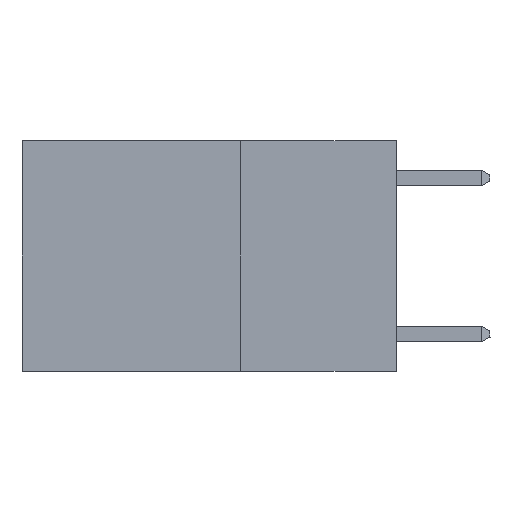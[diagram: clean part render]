
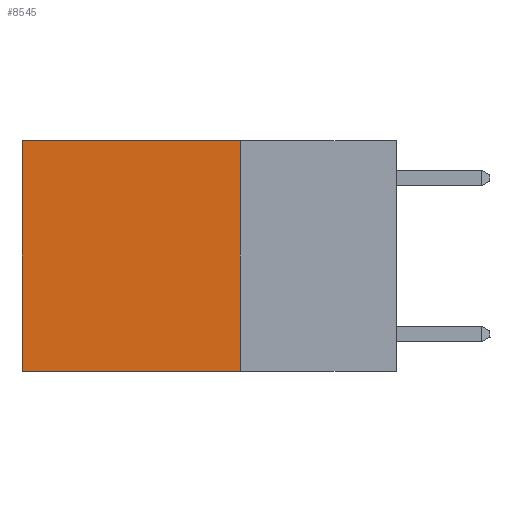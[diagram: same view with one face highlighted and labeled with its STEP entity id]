
A CAD part, left-side view. The second image highlights one B-rep face of the part: STEP entity #8545.
In plain terms, the highlighted planar face has unit normal (-1, 0, 0).
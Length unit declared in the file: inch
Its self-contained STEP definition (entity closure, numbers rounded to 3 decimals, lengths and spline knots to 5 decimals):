
#135 = LINE ( 'NONE', #8784, #15223 ) ;
#398 = CARTESIAN_POINT ( 'NONE',  ( 0.2625, 0.25, 0. ) ) ;
#1139 = CARTESIAN_POINT ( 'NONE',  ( 0.2625, 0.25, -0.37 ) ) ;
#1673 = CARTESIAN_POINT ( 'NONE',  ( 0.2625, 0.25, 0. ) ) ;
#3226 = ORIENTED_EDGE ( 'NONE', *, *, #6788, .T. ) ;
#3668 = DIRECTION ( 'NONE',  ( 0., 0., -1. ) ) ;
#4297 = EDGE_CURVE ( 'NONE', #17747, #10629, #135, .T. ) ;
#4964 = DIRECTION ( 'NONE',  ( 1., 0., 0. ) ) ;
#5156 = PLANE ( 'NONE',  #10344 ) ;
#6229 = CARTESIAN_POINT ( 'NONE',  ( 0.2625, 0.6, -0.37 ) ) ;
#6716 = ORIENTED_EDGE ( 'NONE', *, *, #8570, .F. ) ;
#6788 = EDGE_CURVE ( 'NONE', #15174, #11060, #7929, .T. ) ;
#7489 = EDGE_CURVE ( 'NONE', #11060, #10629, #17031, .T. ) ;
#7929 = LINE ( 'NONE', #1673, #9050 ) ;
#8545 = ADVANCED_FACE ( 'NONE', ( #15701 ), #5156, .F. ) ;
#8570 = EDGE_CURVE ( 'NONE', #15174, #17747, #9753, .T. ) ;
#8784 = CARTESIAN_POINT ( 'NONE',  ( 0.2625, 0.25, -0.37 ) ) ;
#9050 = VECTOR ( 'NONE', #9527, 39.37008 ) ;
#9496 = DIRECTION ( 'NONE',  ( 0., 0., -1. ) ) ;
#9527 = DIRECTION ( 'NONE',  ( 0., 1., 0. ) ) ;
#9539 = DIRECTION ( 'NONE',  ( 0., 0., -1. ) ) ;
#9753 = LINE ( 'NONE', #12835, #13844 ) ;
#10344 = AXIS2_PLACEMENT_3D ( 'NONE', #398, #4964, #3668 ) ;
#10629 = VERTEX_POINT ( 'NONE', #6229 ) ;
#11060 = VERTEX_POINT ( 'NONE', #16993 ) ;
#12835 = CARTESIAN_POINT ( 'NONE',  ( 0.2625, 0.25, 0. ) ) ;
#13844 = VECTOR ( 'NONE', #9539, 39.37008 ) ;
#14232 = ORIENTED_EDGE ( 'NONE', *, *, #7489, .T. ) ;
#14508 = VECTOR ( 'NONE', #9496, 39.37008 ) ;
#14681 = EDGE_LOOP ( 'NONE', ( #14232, #17619, #6716, #3226 ) ) ;
#15174 = VERTEX_POINT ( 'NONE', #19459 ) ;
#15223 = VECTOR ( 'NONE', #16617, 39.37008 ) ;
#15701 = FACE_OUTER_BOUND ( 'NONE', #14681, .T. ) ;
#16617 = DIRECTION ( 'NONE',  ( 0., 1., 0. ) ) ;
#16733 = CARTESIAN_POINT ( 'NONE',  ( 0.2625, 0.6, 0. ) ) ;
#16993 = CARTESIAN_POINT ( 'NONE',  ( 0.2625, 0.6, 0. ) ) ;
#17031 = LINE ( 'NONE', #16733, #14508 ) ;
#17619 = ORIENTED_EDGE ( 'NONE', *, *, #4297, .F. ) ;
#17747 = VERTEX_POINT ( 'NONE', #1139 ) ;
#19459 = CARTESIAN_POINT ( 'NONE',  ( 0.2625, 0.25, 0. ) ) ;
